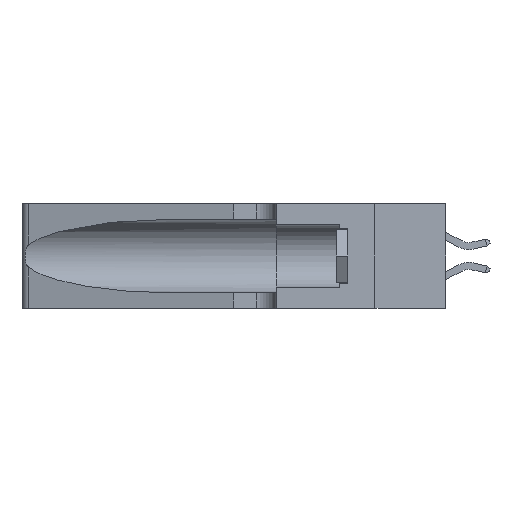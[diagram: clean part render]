
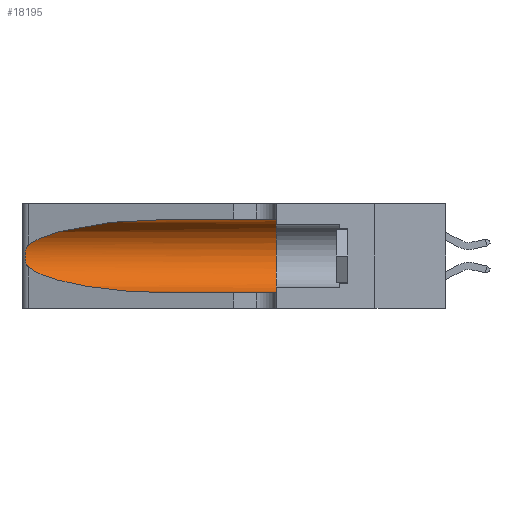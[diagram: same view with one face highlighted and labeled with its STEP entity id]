
A CAD part, left-side view. The second image highlights one B-rep face of the part: STEP entity #18195.
In plain terms, the highlighted cylindrical face has radius 3.308 mm (diameter 6.617 mm), a partial arc.
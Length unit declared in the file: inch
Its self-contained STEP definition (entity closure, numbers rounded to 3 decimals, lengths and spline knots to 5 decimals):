
#326 = CARTESIAN_POINT ( 'NONE',  ( 0.1305, 0.72297, 0.05475 ) ) ;
#1083 = DIRECTION ( 'NONE',  ( 0., -1., 0. ) ) ;
#2570 = CARTESIAN_POINT ( 'NONE',  ( 0.1305, 0.72297, 0.05475 ) ) ;
#3016 = EDGE_CURVE ( 'NONE', #15755, #6408, #27087, .T. ) ;
#3312 = AXIS2_PLACEMENT_3D ( 'NONE', #4514, #22494, #7084 ) ;
#3795 = CARTESIAN_POINT ( 'NONE',  ( 0.26075, 1.23896, 0.178 ) ) ;
#3832 = CARTESIAN_POINT ( 'NONE',  ( 0.25487, 1.22718, 0.22369 ) ) ;
#4235 = CARTESIAN_POINT ( 'NONE',  ( 0.1305, 0.72297, 0.31525 ) ) ;
#4514 = CARTESIAN_POINT ( 'NONE',  ( 0.1305, 0.35, 0.185 ) ) ;
#4841 = VERTEX_POINT ( 'NONE', #9501 ) ;
#6357 = CARTESIAN_POINT ( 'NONE',  ( 0.25856, 1.23593, 0.16098 ) ) ;
#6408 = VERTEX_POINT ( 'NONE', #3832 ) ;
#7084 = DIRECTION ( 'NONE',  ( 0., 0., 1. ) ) ;
#7088 = CARTESIAN_POINT ( 'NONE',  ( 0.25487, 1.22718, 0.22369 ) ) ;
#8708 = VERTEX_POINT ( 'NONE', #10934 ) ;
#8950 = CARTESIAN_POINT ( 'NONE',  ( 0.25639, 1.23186, 0.15144 ) ) ;
#8968 = ORIENTED_EDGE ( 'NONE', *, *, #33253, .F. ) ;
#9036 = EDGE_CURVE ( 'NONE', #8708, #4841, #31907, .T. ) ;
#9501 = CARTESIAN_POINT ( 'NONE',  ( 0.1305, 0.35, 0.05475 ) ) ;
#9600 = CARTESIAN_POINT ( 'NONE',  ( 0.25487, 1.22718, 0.14631 ) ) ;
#9780 = CARTESIAN_POINT ( 'NONE',  ( 0.25555, 1.22994, 0.2215 ) ) ;
#10266 = LINE ( 'NONE', #25497, #16341 ) ;
#10609 = CARTESIAN_POINT ( 'NONE',  ( 0.1305, 1.61858, 0.05475 ) ) ;
#10934 = CARTESIAN_POINT ( 'NONE',  ( 0.1305, 0.35, 0.31525 ) ) ;
#11020 = EDGE_CURVE ( 'NONE', #6408, #23752, #30564, .T. ) ;
#11557 = CARTESIAN_POINT ( 'NONE',  ( 0.25487, 1.22718, 0.14631 ) ) ;
#12679 =( BOUNDED_CURVE ( )  B_SPLINE_CURVE ( 3, ( #30691, #25647, #18041, #2570 ),
 .UNSPECIFIED., .F., .T. ) 
 B_SPLINE_CURVE_WITH_KNOTS ( ( 4, 4 ),
 ( 3.44316, 4.71239 ),
 .UNSPECIFIED. ) 
 CURVE ( )  GEOMETRIC_REPRESENTATION_ITEM ( )  RATIONAL_B_SPLINE_CURVE ( ( 1., 0.87, 0.87, 1. ) ) 
 REPRESENTATION_ITEM ( '' )  );
#12921 = CARTESIAN_POINT ( 'NONE',  ( 0.25487, 1.22718, 0.22369 ) ) ;
#13210 = DIRECTION ( 'NONE',  ( 0., -1., 0. ) ) ;
#13955 = EDGE_CURVE ( 'NONE', #23752, #32753, #12679, .T. ) ;
#14129 = ORIENTED_EDGE ( 'NONE', *, *, #11020, .T. ) ;
#14335 = AXIS2_PLACEMENT_3D ( 'NONE', #24220, #1083, #21533 ) ;
#14995 = CARTESIAN_POINT ( 'NONE',  ( 0.25639, 1.23184, 0.21858 ) ) ;
#15325 = DIRECTION ( 'NONE',  ( 0., -1., 0. ) ) ;
#15755 = VERTEX_POINT ( 'NONE', #4235 ) ;
#16341 = VECTOR ( 'NONE', #15325, 39.37008 ) ;
#17103 = CYLINDRICAL_SURFACE ( 'NONE', #14335, 0.13025 ) ;
#17443 = EDGE_LOOP ( 'NONE', ( #30559, #14129, #22207, #19411, #23851, #8968 ) ) ;
#17574 = CARTESIAN_POINT ( 'NONE',  ( 0.25854, 1.2359, 0.20912 ) ) ;
#17976 = CARTESIAN_POINT ( 'NONE',  ( 0.18966, 0.96281, 0.31525 ) ) ;
#18041 = CARTESIAN_POINT ( 'NONE',  ( 0.18966, 0.96281, 0.05475 ) ) ;
#18195 = ADVANCED_FACE ( 'NONE', ( #33100 ), #17103, .F. ) ;
#18661 = EDGE_CURVE ( 'NONE', #32753, #4841, #31916, .T. ) ;
#19214 = CARTESIAN_POINT ( 'NONE',  ( 0.26075, 1.23896, 0.19203 ) ) ;
#19411 = ORIENTED_EDGE ( 'NONE', *, *, #18661, .T. ) ;
#21533 = DIRECTION ( 'NONE',  ( 0., 0., -1. ) ) ;
#21771 = CARTESIAN_POINT ( 'NONE',  ( 0.26017, 1.23833, 0.17102 ) ) ;
#22207 = ORIENTED_EDGE ( 'NONE', *, *, #13955, .T. ) ;
#22494 = DIRECTION ( 'NONE',  ( 0., 1., 0. ) ) ;
#23115 = CARTESIAN_POINT ( 'NONE',  ( 0.2373, 1.15595, 0.28018 ) ) ;
#23752 = VERTEX_POINT ( 'NONE', #9600 ) ;
#23851 = ORIENTED_EDGE ( 'NONE', *, *, #9036, .F. ) ;
#24220 = CARTESIAN_POINT ( 'NONE',  ( 0.1305, 1.61858, 0.185 ) ) ;
#24343 = CARTESIAN_POINT ( 'NONE',  ( 0.25789, 1.23486, 0.15765 ) ) ;
#25128 = VECTOR ( 'NONE', #13210, 39.37008 ) ;
#25497 = CARTESIAN_POINT ( 'NONE',  ( 0.1305, 1.61858, 0.31525 ) ) ;
#25647 = CARTESIAN_POINT ( 'NONE',  ( 0.2373, 1.15595, 0.08982 ) ) ;
#26945 = CARTESIAN_POINT ( 'NONE',  ( 0.25555, 1.22993, 0.14849 ) ) ;
#27087 =( BOUNDED_CURVE ( )  B_SPLINE_CURVE ( 3, ( #28270, #17976, #23115, #12921 ),
 .UNSPECIFIED., .F., .T. ) 
 B_SPLINE_CURVE_WITH_KNOTS ( ( 4, 4 ),
 ( 1.5708, 2.84003 ),
 .UNSPECIFIED. ) 
 CURVE ( )  GEOMETRIC_REPRESENTATION_ITEM ( )  RATIONAL_B_SPLINE_CURVE ( ( 1., 0.87, 0.87, 1. ) ) 
 REPRESENTATION_ITEM ( '' )  );
#27802 = CARTESIAN_POINT ( 'NONE',  ( 0.26018, 1.23835, 0.19895 ) ) ;
#28270 = CARTESIAN_POINT ( 'NONE',  ( 0.1305, 0.72297, 0.31525 ) ) ;
#30559 = ORIENTED_EDGE ( 'NONE', *, *, #3016, .T. ) ;
#30564 = B_SPLINE_CURVE_WITH_KNOTS ( 'NONE', 3,
 ( #7088, #9780, #14995, #32887, #17574, #27802, #19214, #3795, #21771, #6357, #24343, #8950, #26945, #11557 ),
 .UNSPECIFIED., .F., .F.,
 ( 4, 2, 2, 2, 2, 2, 4 ),
 ( 0., 0.00027, 0.00053, 0.00107, 0.0016, 0.00187, 0.00214 ),
 .UNSPECIFIED. ) ;
#30691 = CARTESIAN_POINT ( 'NONE',  ( 0.25487, 1.22718, 0.14631 ) ) ;
#31907 = CIRCLE ( 'NONE', #3312, 0.13025 ) ;
#31916 = LINE ( 'NONE', #10609, #25128 ) ;
#32753 = VERTEX_POINT ( 'NONE', #326 ) ;
#32887 = CARTESIAN_POINT ( 'NONE',  ( 0.25787, 1.23484, 0.2124 ) ) ;
#33100 = FACE_OUTER_BOUND ( 'NONE', #17443, .T. ) ;
#33253 = EDGE_CURVE ( 'NONE', #15755, #8708, #10266, .T. ) ;
